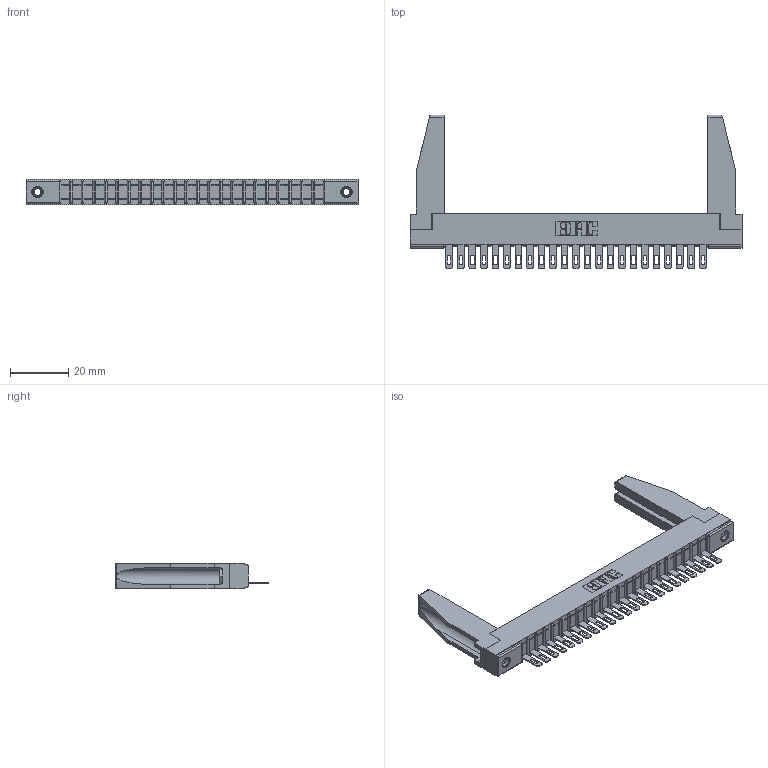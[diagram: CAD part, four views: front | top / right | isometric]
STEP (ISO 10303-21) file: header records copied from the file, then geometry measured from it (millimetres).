
FILE_DESCRIPTION (( 'STEP AP203' ), '1' );
FILE_NAME ('357-023-405-178.STEP', '2020-10-01T09:42:52', ( '' ), ( '' ), 'SwSTEP 2.0', 'SolidWorks 2020', '' );
FILE_SCHEMA (( 'CONFIG_CONTROL_DESIGN' ));
Length unit declared in the file: inch
Products named in the file (5): 307-290-001_505; 307 Part_.156 Dia Mounting Holes; 307-220-078; 345-250-001_345-250-001-102; 357-023-405-178
Assembly tree (28 placements, depth 2):
  357-023-405-178
    307 Part_.156 Dia Mounting Holes
    307-290-001_505  x23
    307-220-078  x2
    345-250-001_345-250-001-102  x2
Bounding box: 114.15 x 52.88 x 8.71 mm (x, y, z)
Volume: 11228.9 mm3; surface area: 15269.8 mm2
Topology: 28 solids, 28 shells, 1560 faces, 4379 edges, 2814 vertices
Faces by surface type: plane 982, cylinder 514, sphere 48, cone 12, torus 4
Entity records: 24473 total; most frequent: CARTESIAN_POINT 4114, ORIENTED_EDGE 4056, DIRECTION 3970, EDGE_CURVE 2028, VECTOR 1550, LINE 1550, VERTEX_POINT 1312, AXIS2_PLACEMENT_3D 1210
